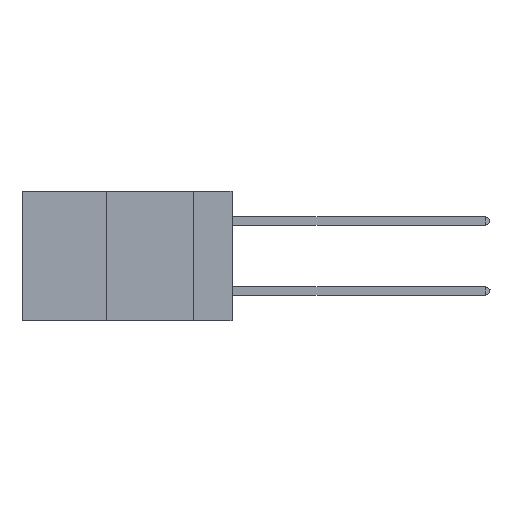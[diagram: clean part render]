
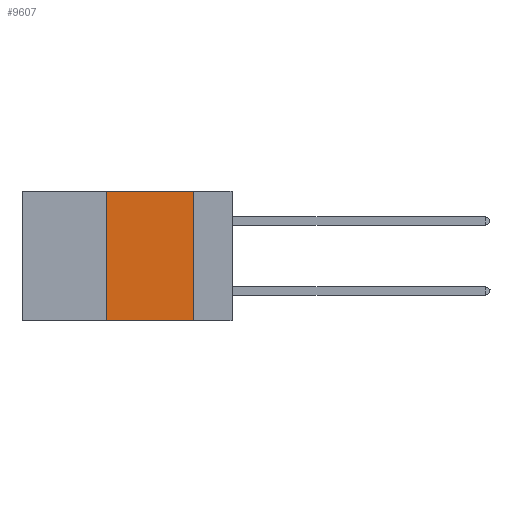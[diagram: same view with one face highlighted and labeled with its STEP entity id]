
A CAD part, left-side view. The second image highlights one B-rep face of the part: STEP entity #9607.
In plain terms, the highlighted planar face has unit normal (-1, 0, 0).
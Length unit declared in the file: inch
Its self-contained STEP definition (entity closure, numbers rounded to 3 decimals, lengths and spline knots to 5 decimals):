
#845 = EDGE_LOOP ( 'NONE', ( #9441, #7613, #14068, #15110 ) ) ;
#1241 = CARTESIAN_POINT ( 'NONE',  ( 0., 0.36, -0.37 ) ) ;
#3251 = EDGE_CURVE ( 'NONE', #10018, #23713, #25346, .T. ) ;
#4041 = DIRECTION ( 'NONE',  ( 0., 0., -1. ) ) ;
#4497 = DIRECTION ( 'NONE',  ( 1., 0., 0. ) ) ;
#4707 = VERTEX_POINT ( 'NONE', #25692 ) ;
#7129 = VECTOR ( 'NONE', #8167, 39.37008 ) ;
#7613 = ORIENTED_EDGE ( 'NONE', *, *, #18759, .F. ) ;
#8167 = DIRECTION ( 'NONE',  ( 0., -1., 0. ) ) ;
#8184 = LINE ( 'NONE', #10349, #20557 ) ;
#9441 = ORIENTED_EDGE ( 'NONE', *, *, #11353, .F. ) ;
#9490 = EDGE_CURVE ( 'NONE', #10018, #9571, #8184, .T. ) ;
#9571 = VERTEX_POINT ( 'NONE', #12809 ) ;
#9607 = ADVANCED_FACE ( 'NONE', ( #25201 ), #20466, .F. ) ;
#10018 = VERTEX_POINT ( 'NONE', #1241 ) ;
#10174 = LINE ( 'NONE', #17507, #7129 ) ;
#10349 = CARTESIAN_POINT ( 'NONE',  ( 0., 0.36, 0. ) ) ;
#11353 = EDGE_CURVE ( 'NONE', #4707, #23713, #20426, .T. ) ;
#12256 = AXIS2_PLACEMENT_3D ( 'NONE', #20621, #4497, #4041 ) ;
#12809 = CARTESIAN_POINT ( 'NONE',  ( 0., 0.36, 0. ) ) ;
#13820 = DIRECTION ( 'NONE',  ( 0., 0., -1. ) ) ;
#14068 = ORIENTED_EDGE ( 'NONE', *, *, #9490, .F. ) ;
#14922 = DIRECTION ( 'NONE',  ( 0., 0., 1. ) ) ;
#15110 = ORIENTED_EDGE ( 'NONE', *, *, #3251, .T. ) ;
#17507 = CARTESIAN_POINT ( 'NONE',  ( 0., 0.6, 0. ) ) ;
#17654 = VECTOR ( 'NONE', #13820, 39.37008 ) ;
#18759 = EDGE_CURVE ( 'NONE', #9571, #4707, #10174, .T. ) ;
#20161 = DIRECTION ( 'NONE',  ( 0., -1., 0. ) ) ;
#20426 = LINE ( 'NONE', #25167, #17654 ) ;
#20466 = PLANE ( 'NONE',  #12256 ) ;
#20557 = VECTOR ( 'NONE', #14922, 39.37008 ) ;
#20621 = CARTESIAN_POINT ( 'NONE',  ( 0., 0.6, 0. ) ) ;
#22442 = CARTESIAN_POINT ( 'NONE',  ( 0., 0.6, -0.37 ) ) ;
#23282 = VECTOR ( 'NONE', #20161, 39.37008 ) ;
#23713 = VERTEX_POINT ( 'NONE', #23868 ) ;
#23868 = CARTESIAN_POINT ( 'NONE',  ( 0., 0.11, -0.37 ) ) ;
#25167 = CARTESIAN_POINT ( 'NONE',  ( 0., 0.11, 0. ) ) ;
#25201 = FACE_OUTER_BOUND ( 'NONE', #845, .T. ) ;
#25346 = LINE ( 'NONE', #22442, #23282 ) ;
#25692 = CARTESIAN_POINT ( 'NONE',  ( 0., 0.11, 0. ) ) ;
